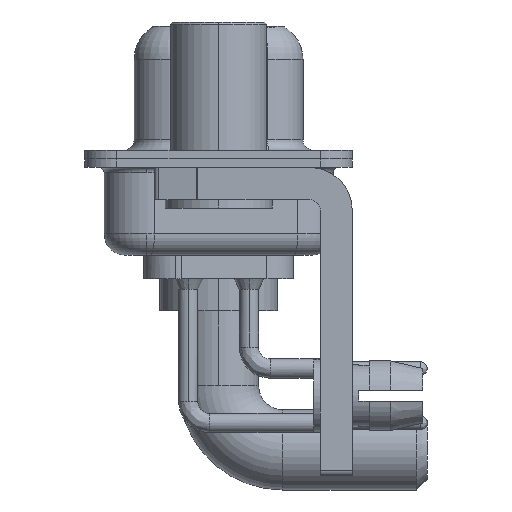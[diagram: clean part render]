
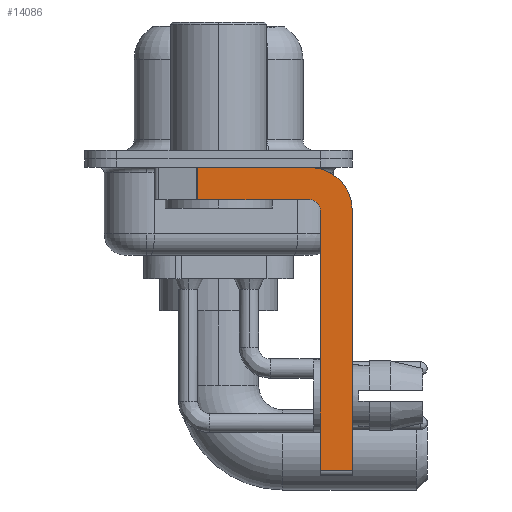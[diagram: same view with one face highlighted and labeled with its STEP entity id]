
A CAD part, left-side view. The second image highlights one B-rep face of the part: STEP entity #14086.
In plain terms, the highlighted planar face has unit normal (-1, 0, 0).
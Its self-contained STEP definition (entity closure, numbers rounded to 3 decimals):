
#301 = VERTEX_POINT ( 'NONE', #11690 ) ;
#326 = VERTEX_POINT ( 'NONE', #7406 ) ;
#336 = CARTESIAN_POINT ( 'NONE',  ( -2.9, 0.978, -0.4 ) ) ;
#558 = EDGE_CURVE ( 'NONE', #15413, #12556, #16435, .T. ) ;
#1144 = EDGE_LOOP ( 'NONE', ( #18764, #15789, #1662, #8588, #10779, #1303, #18390, #2280 ) ) ;
#1262 = CARTESIAN_POINT ( 'NONE',  ( -2.9, 0.978, -1.9 ) ) ;
#1303 = ORIENTED_EDGE ( 'NONE', *, *, #14371, .T. ) ;
#1662 = ORIENTED_EDGE ( 'NONE', *, *, #12982, .F. ) ;
#1870 = LINE ( 'NONE', #15966, #20573 ) ;
#2280 = ORIENTED_EDGE ( 'NONE', *, *, #7325, .F. ) ;
#3156 = DIRECTION ( 'NONE',  ( 0., 0., -1. ) ) ;
#3196 = CARTESIAN_POINT ( 'NONE',  ( -2.9, 3., -0.4 ) ) ;
#3697 = VECTOR ( 'NONE', #14464, 1000. ) ;
#3852 = LINE ( 'NONE', #19677, #3697 ) ;
#4648 = CARTESIAN_POINT ( 'NONE',  ( -2.9, -6.25, -14.55 ) ) ;
#4668 = DIRECTION ( 'NONE',  ( 1., 0., 0. ) ) ;
#4869 = DIRECTION ( 'NONE',  ( 0., 0., 1. ) ) ;
#5168 = DIRECTION ( 'NONE',  ( -1., 0., 0. ) ) ;
#5454 = DIRECTION ( 'NONE',  ( 0., 1., 0. ) ) ;
#7021 = DIRECTION ( 'NONE',  ( 0., 0., 1. ) ) ;
#7325 = EDGE_CURVE ( 'NONE', #326, #301, #15184, .T. ) ;
#7406 = CARTESIAN_POINT ( 'NONE',  ( -2.9, -4.25, -0.4 ) ) ;
#7656 = CARTESIAN_POINT ( 'NONE',  ( -2.9, 0.978, -1.9 ) ) ;
#7810 = VERTEX_POINT ( 'NONE', #4648 ) ;
#8132 = LINE ( 'NONE', #13324, #14531 ) ;
#8576 = AXIS2_PLACEMENT_3D ( 'NONE', #20893, #5168, #7021 ) ;
#8588 = ORIENTED_EDGE ( 'NONE', *, *, #18012, .F. ) ;
#8742 = LINE ( 'NONE', #3196, #12551 ) ;
#8839 = EDGE_CURVE ( 'NONE', #22707, #17769, #8132, .T. ) ;
#8966 = VERTEX_POINT ( 'NONE', #15840 ) ;
#9966 = AXIS2_PLACEMENT_3D ( 'NONE', #20511, #4668, #3156 ) ;
#10608 = LINE ( 'NONE', #11998, #20599 ) ;
#10779 = ORIENTED_EDGE ( 'NONE', *, *, #8839, .F. ) ;
#11690 = CARTESIAN_POINT ( 'NONE',  ( -2.9, -6.25, -2.4 ) ) ;
#11729 = DIRECTION ( 'NONE',  ( 0., 0., -1. ) ) ;
#11830 = CARTESIAN_POINT ( 'NONE',  ( -2.9, -4.25, -2.4 ) ) ;
#11998 = CARTESIAN_POINT ( 'NONE',  ( -2.9, -6.25, -2.4 ) ) ;
#12551 = VECTOR ( 'NONE', #14282, 1000. ) ;
#12556 = VERTEX_POINT ( 'NONE', #1262 ) ;
#12982 = EDGE_CURVE ( 'NONE', #8966, #12556, #1870, .T. ) ;
#13324 = CARTESIAN_POINT ( 'NONE',  ( -2.9, -4.75, -14.8 ) ) ;
#13837 = EDGE_CURVE ( 'NONE', #301, #7810, #10608, .T. ) ;
#13845 = DIRECTION ( 'NONE',  ( 0., 0., -1. ) ) ;
#14086 = ADVANCED_FACE ( 'NONE', ( #22343 ), #20834, .F. ) ;
#14102 = CIRCLE ( 'NONE', #8576, 0.5 ) ;
#14282 = DIRECTION ( 'NONE',  ( 0., -1., 0. ) ) ;
#14371 = EDGE_CURVE ( 'NONE', #22707, #7810, #3852, .T. ) ;
#14464 = DIRECTION ( 'NONE',  ( 0., -1., 0. ) ) ;
#14531 = VECTOR ( 'NONE', #4869, 1000. ) ;
#15184 = CIRCLE ( 'NONE', #18868, 2. ) ;
#15413 = VERTEX_POINT ( 'NONE', #336 ) ;
#15789 = ORIENTED_EDGE ( 'NONE', *, *, #558, .T. ) ;
#15840 = CARTESIAN_POINT ( 'NONE',  ( -2.9, -4.25, -1.9 ) ) ;
#15966 = CARTESIAN_POINT ( 'NONE',  ( -2.9, -4.25, -1.9 ) ) ;
#16435 = LINE ( 'NONE', #7656, #21285 ) ;
#17109 = CARTESIAN_POINT ( 'NONE',  ( -2.9, -4.75, -14.55 ) ) ;
#17769 = VERTEX_POINT ( 'NONE', #20457 ) ;
#18012 = EDGE_CURVE ( 'NONE', #17769, #8966, #14102, .T. ) ;
#18390 = ORIENTED_EDGE ( 'NONE', *, *, #13837, .F. ) ;
#18764 = ORIENTED_EDGE ( 'NONE', *, *, #19872, .F. ) ;
#18868 = AXIS2_PLACEMENT_3D ( 'NONE', #11830, #20184, #11729 ) ;
#19677 = CARTESIAN_POINT ( 'NONE',  ( -2.9, -4.25, -14.55 ) ) ;
#19872 = EDGE_CURVE ( 'NONE', #15413, #326, #8742, .T. ) ;
#20184 = DIRECTION ( 'NONE',  ( 1., 0., 0. ) ) ;
#20457 = CARTESIAN_POINT ( 'NONE',  ( -2.9, -4.75, -2.4 ) ) ;
#20511 = CARTESIAN_POINT ( 'NONE',  ( -2.9, -4.25, -2.4 ) ) ;
#20573 = VECTOR ( 'NONE', #5454, 1000. ) ;
#20599 = VECTOR ( 'NONE', #13845, 1000. ) ;
#20834 = PLANE ( 'NONE',  #9966 ) ;
#20893 = CARTESIAN_POINT ( 'NONE',  ( -2.9, -4.25, -2.4 ) ) ;
#21285 = VECTOR ( 'NONE', #21737, 1000. ) ;
#21737 = DIRECTION ( 'NONE',  ( 0., 0., -1. ) ) ;
#22343 = FACE_OUTER_BOUND ( 'NONE', #1144, .T. ) ;
#22707 = VERTEX_POINT ( 'NONE', #17109 ) ;
